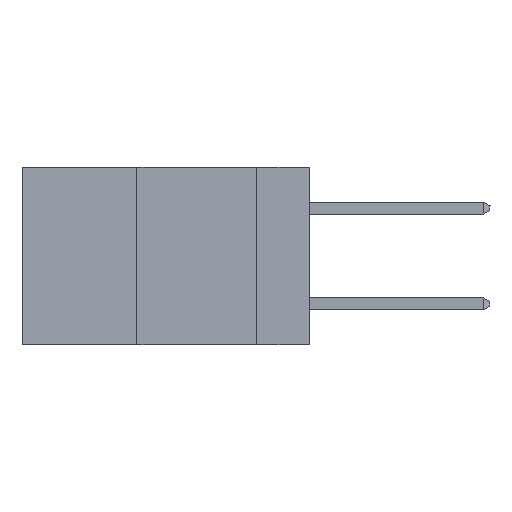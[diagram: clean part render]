
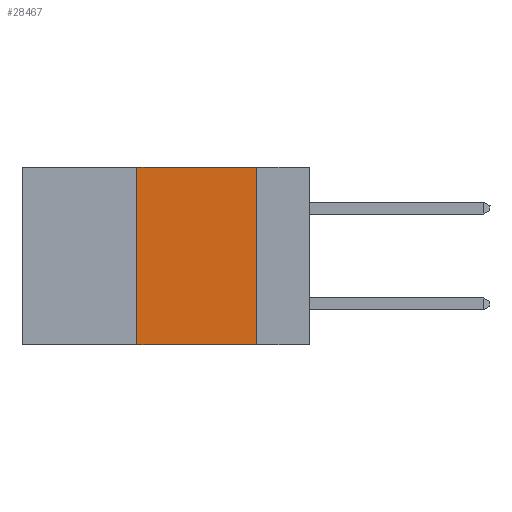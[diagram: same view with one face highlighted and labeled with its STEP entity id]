
A CAD part, left-side view. The second image highlights one B-rep face of the part: STEP entity #28467.
In plain terms, the highlighted planar face has unit normal (-1, 0, 0).
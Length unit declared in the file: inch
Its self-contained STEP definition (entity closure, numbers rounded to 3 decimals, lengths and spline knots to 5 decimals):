
#988 = EDGE_CURVE ( 'NONE', #7278, #18893, #28972, .T. ) ;
#1345 = PLANE ( 'NONE',  #21951 ) ;
#1625 = DIRECTION ( 'NONE',  ( 0., 0., -1. ) ) ;
#2251 = CARTESIAN_POINT ( 'NONE',  ( 0., 0.36, 0. ) ) ;
#2782 = ORIENTED_EDGE ( 'NONE', *, *, #13993, .T. ) ;
#3645 = CARTESIAN_POINT ( 'NONE',  ( 0., 0.11, 0. ) ) ;
#4029 = CARTESIAN_POINT ( 'NONE',  ( 0., 0.36, 0. ) ) ;
#6422 = EDGE_CURVE ( 'NONE', #10885, #15065, #9572, .T. ) ;
#7278 = VERTEX_POINT ( 'NONE', #16265 ) ;
#8236 = CARTESIAN_POINT ( 'NONE',  ( 0., 0.6, 0. ) ) ;
#8835 = CARTESIAN_POINT ( 'NONE',  ( 0., 0.11, -0.37 ) ) ;
#8880 = ORIENTED_EDGE ( 'NONE', *, *, #20041, .F. ) ;
#9282 = VECTOR ( 'NONE', #21947, 39.37008 ) ;
#9572 = LINE ( 'NONE', #25154, #27479 ) ;
#10885 = VERTEX_POINT ( 'NONE', #3645 ) ;
#12892 = ORIENTED_EDGE ( 'NONE', *, *, #988, .F. ) ;
#13993 = EDGE_CURVE ( 'NONE', #7278, #15065, #28781, .T. ) ;
#14656 = CARTESIAN_POINT ( 'NONE',  ( 0., 0.6, -0.37 ) ) ;
#14873 = LINE ( 'NONE', #19688, #9282 ) ;
#15065 = VERTEX_POINT ( 'NONE', #8835 ) ;
#16265 = CARTESIAN_POINT ( 'NONE',  ( 0., 0.36, -0.37 ) ) ;
#16951 = FACE_OUTER_BOUND ( 'NONE', #17803, .T. ) ;
#17803 = EDGE_LOOP ( 'NONE', ( #25622, #8880, #12892, #2782 ) ) ;
#18725 = DIRECTION ( 'NONE',  ( 0., 0., -1. ) ) ;
#18893 = VERTEX_POINT ( 'NONE', #2251 ) ;
#19688 = CARTESIAN_POINT ( 'NONE',  ( 0., 0.6, 0. ) ) ;
#20041 = EDGE_CURVE ( 'NONE', #18893, #10885, #14873, .T. ) ;
#21719 = DIRECTION ( 'NONE',  ( 0., -1., 0. ) ) ;
#21947 = DIRECTION ( 'NONE',  ( 0., -1., 0. ) ) ;
#21951 = AXIS2_PLACEMENT_3D ( 'NONE', #8236, #24293, #1625 ) ;
#24293 = DIRECTION ( 'NONE',  ( 1., 0., 0. ) ) ;
#24463 = DIRECTION ( 'NONE',  ( 0., 0., 1. ) ) ;
#25154 = CARTESIAN_POINT ( 'NONE',  ( 0., 0.11, 0. ) ) ;
#25311 = VECTOR ( 'NONE', #21719, 39.37008 ) ;
#25622 = ORIENTED_EDGE ( 'NONE', *, *, #6422, .F. ) ;
#27479 = VECTOR ( 'NONE', #18725, 39.37008 ) ;
#28467 = ADVANCED_FACE ( 'NONE', ( #16951 ), #1345, .F. ) ;
#28545 = VECTOR ( 'NONE', #24463, 39.37008 ) ;
#28781 = LINE ( 'NONE', #14656, #25311 ) ;
#28972 = LINE ( 'NONE', #4029, #28545 ) ;
